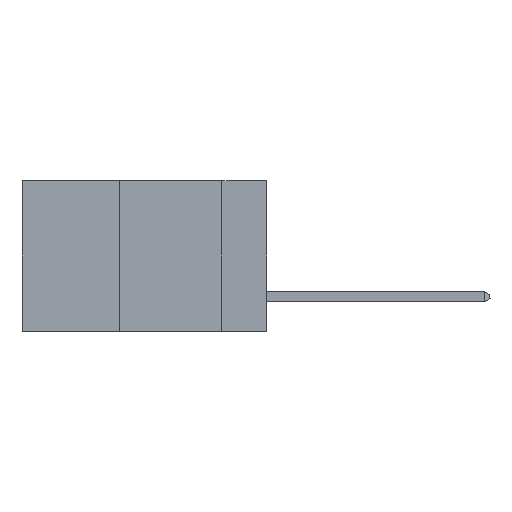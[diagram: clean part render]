
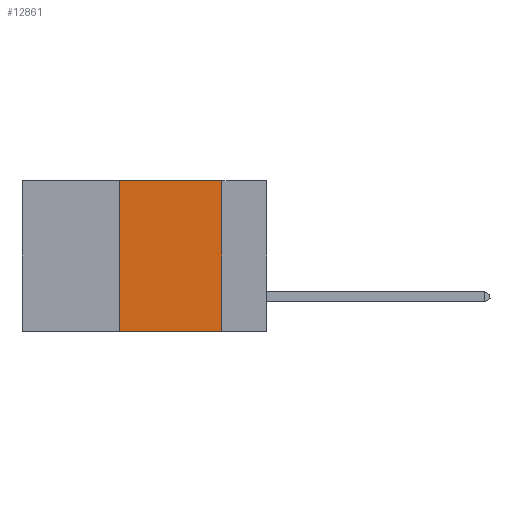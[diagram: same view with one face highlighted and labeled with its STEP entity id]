
A CAD part, left-side view. The second image highlights one B-rep face of the part: STEP entity #12861.
In plain terms, the highlighted planar face has unit normal (-1, 0, 0).
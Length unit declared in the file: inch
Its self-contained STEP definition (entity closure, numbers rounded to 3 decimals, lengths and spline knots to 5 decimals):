
#840 = VERTEX_POINT ( 'NONE', #847 ) ;
#847 = CARTESIAN_POINT ( 'NONE',  ( 0., 0.36, -0.37 ) ) ;
#2003 = VERTEX_POINT ( 'NONE', #7999 ) ;
#3243 = ORIENTED_EDGE ( 'NONE', *, *, #19762, .F. ) ;
#4528 = LINE ( 'NONE', #6436, #8497 ) ;
#5558 = LINE ( 'NONE', #14548, #17040 ) ;
#5764 = CARTESIAN_POINT ( 'NONE',  ( 0., 0.11, 0. ) ) ;
#6195 = VERTEX_POINT ( 'NONE', #15128 ) ;
#6436 = CARTESIAN_POINT ( 'NONE',  ( 0., 0.36, 0. ) ) ;
#6925 = PLANE ( 'NONE',  #10316 ) ;
#6945 = DIRECTION ( 'NONE',  ( 0., 0., -1. ) ) ;
#7978 = VECTOR ( 'NONE', #21005, 39.37008 ) ;
#7999 = CARTESIAN_POINT ( 'NONE',  ( 0., 0.36, 0. ) ) ;
#8497 = VECTOR ( 'NONE', #23450, 39.37008 ) ;
#8705 = DIRECTION ( 'NONE',  ( 1., 0., 0. ) ) ;
#10137 = EDGE_LOOP ( 'NONE', ( #12936, #15424, #3243, #13780 ) ) ;
#10316 = AXIS2_PLACEMENT_3D ( 'NONE', #20414, #8705, #20327 ) ;
#11973 = CARTESIAN_POINT ( 'NONE',  ( 0., 0.6, 0. ) ) ;
#12775 = FACE_OUTER_BOUND ( 'NONE', #10137, .T. ) ;
#12861 = ADVANCED_FACE ( 'NONE', ( #12775 ), #6925, .F. ) ;
#12936 = ORIENTED_EDGE ( 'NONE', *, *, #23015, .F. ) ;
#13085 = LINE ( 'NONE', #13306, #7978 ) ;
#13306 = CARTESIAN_POINT ( 'NONE',  ( 0., 0.6, -0.37 ) ) ;
#13780 = ORIENTED_EDGE ( 'NONE', *, *, #23536, .T. ) ;
#14548 = CARTESIAN_POINT ( 'NONE',  ( 0., 0.11, 0. ) ) ;
#14942 = EDGE_CURVE ( 'NONE', #2003, #18287, #18995, .T. ) ;
#15128 = CARTESIAN_POINT ( 'NONE',  ( 0., 0.11, -0.37 ) ) ;
#15424 = ORIENTED_EDGE ( 'NONE', *, *, #14942, .F. ) ;
#17040 = VECTOR ( 'NONE', #6945, 39.37008 ) ;
#17208 = VECTOR ( 'NONE', #23335, 39.37008 ) ;
#18287 = VERTEX_POINT ( 'NONE', #5764 ) ;
#18995 = LINE ( 'NONE', #11973, #17208 ) ;
#19762 = EDGE_CURVE ( 'NONE', #840, #2003, #4528, .T. ) ;
#20327 = DIRECTION ( 'NONE',  ( 0., 0., -1. ) ) ;
#20414 = CARTESIAN_POINT ( 'NONE',  ( 0., 0.6, 0. ) ) ;
#21005 = DIRECTION ( 'NONE',  ( 0., -1., 0. ) ) ;
#23015 = EDGE_CURVE ( 'NONE', #18287, #6195, #5558, .T. ) ;
#23335 = DIRECTION ( 'NONE',  ( 0., -1., 0. ) ) ;
#23450 = DIRECTION ( 'NONE',  ( 0., 0., 1. ) ) ;
#23536 = EDGE_CURVE ( 'NONE', #840, #6195, #13085, .T. ) ;
